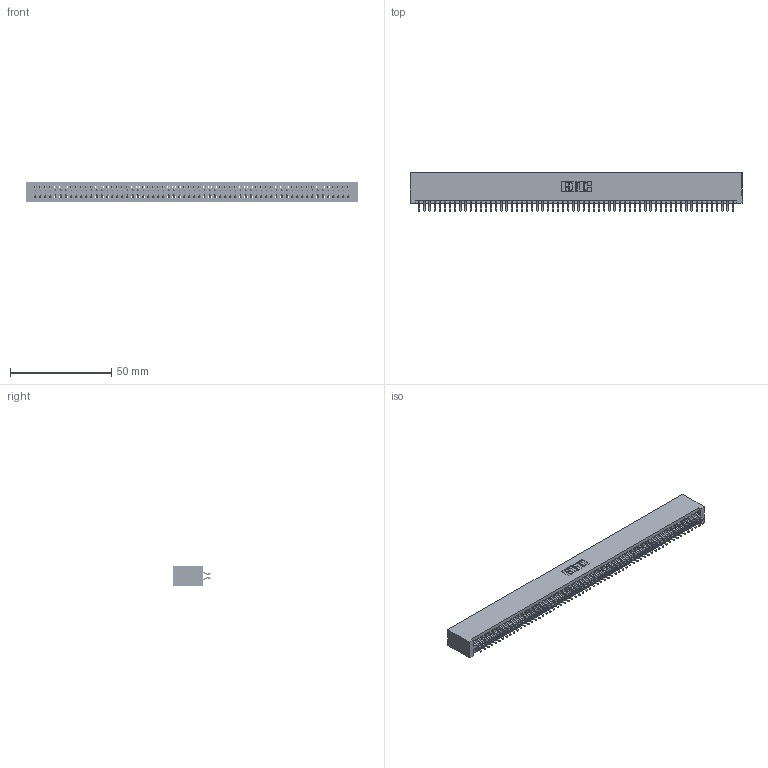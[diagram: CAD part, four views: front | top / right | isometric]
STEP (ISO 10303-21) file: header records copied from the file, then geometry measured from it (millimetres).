
FILE_DESCRIPTION (( 'STEP AP203' ), '1' );
FILE_NAME ('345-124-556-201.STEP', '2018-10-19T10:57:53', ( '' ), ( '' ), 'SwSTEP 2.0', 'SolidWorks 2016', '' );
FILE_SCHEMA (( 'CONFIG_CONTROL_DESIGN' ));
Length unit declared in the file: inch
Products named in the file (3): 345-124-556-201; 345-292-001_556 Tail; 345 Part_No Mounting Lugs
Assembly tree (125 placements, depth 2):
  345-124-556-201
    345 Part_No Mounting Lugs
    345-292-001_556 Tail  x124
Bounding box: 164.08 x 19.24 x 9.4 mm (x, y, z)
Volume: 16735.9 mm3; surface area: 25320.6 mm2
Topology: 125 solids, 125 shells, 7062 faces, 21025 edges, 13850 vertices
Faces by surface type: plane 4664, cylinder 2398
Entity records: 45897 total; most frequent: CARTESIAN_POINT 7688, ORIENTED_EDGE 7610, DIRECTION 6737, EDGE_CURVE 3805, LINE 3425, VECTOR 3425, VERTEX_POINT 2534, AXIS2_PLACEMENT_3D 1656
